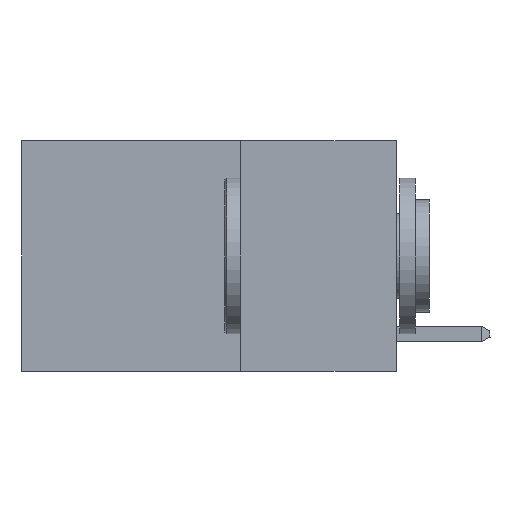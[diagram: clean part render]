
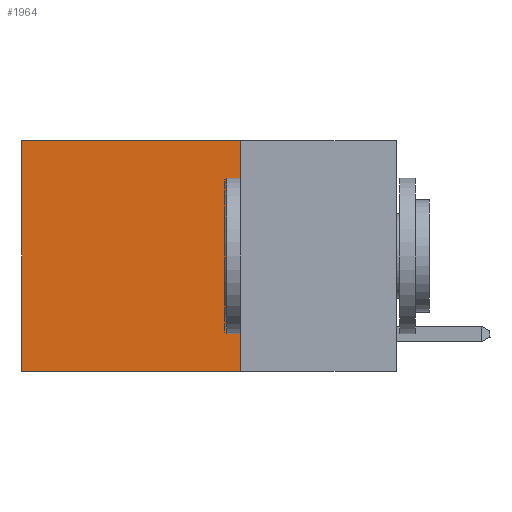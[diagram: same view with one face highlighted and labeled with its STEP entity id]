
A CAD part, left-side view. The second image highlights one B-rep face of the part: STEP entity #1964.
In plain terms, the highlighted planar face has unit normal (-1, 0, 0).
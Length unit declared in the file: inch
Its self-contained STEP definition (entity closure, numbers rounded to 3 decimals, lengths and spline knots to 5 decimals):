
#124 = LINE ( 'NONE', #7129, #6076 ) ;
#725 = VECTOR ( 'NONE', #1364, 39.37008 ) ;
#837 = EDGE_CURVE ( 'NONE', #999, #3835, #2540, .T. ) ;
#895 = DIRECTION ( 'NONE',  ( 0., 0., -1. ) ) ;
#999 = VERTEX_POINT ( 'NONE', #2601 ) ;
#1364 = DIRECTION ( 'NONE',  ( 0., 1., 0. ) ) ;
#1964 = ADVANCED_FACE ( 'NONE', ( #4877 ), #3511, .F. ) ;
#2136 = CARTESIAN_POINT ( 'NONE',  ( 0.2625, 0.25, -0.37 ) ) ;
#2264 = VERTEX_POINT ( 'NONE', #3410 ) ;
#2334 = CARTESIAN_POINT ( 'NONE',  ( 0.2625, 0.25, 0. ) ) ;
#2442 = DIRECTION ( 'NONE',  ( 0., 1., 0. ) ) ;
#2540 = LINE ( 'NONE', #2334, #4622 ) ;
#2601 = CARTESIAN_POINT ( 'NONE',  ( 0.2625, 0.25, 0. ) ) ;
#3062 = EDGE_CURVE ( 'NONE', #999, #2264, #9534, .T. ) ;
#3334 = CARTESIAN_POINT ( 'NONE',  ( 0.2625, 0.25, 0. ) ) ;
#3410 = CARTESIAN_POINT ( 'NONE',  ( 0.2625, 0.6, 0. ) ) ;
#3511 = PLANE ( 'NONE',  #5679 ) ;
#3623 = CARTESIAN_POINT ( 'NONE',  ( 0.2625, 0.6, -0.37 ) ) ;
#3731 = ORIENTED_EDGE ( 'NONE', *, *, #4255, .F. ) ;
#3835 = VERTEX_POINT ( 'NONE', #9492 ) ;
#3867 = ORIENTED_EDGE ( 'NONE', *, *, #837, .F. ) ;
#4100 = DIRECTION ( 'NONE',  ( 0., 0., -1. ) ) ;
#4255 = EDGE_CURVE ( 'NONE', #3835, #6592, #6164, .T. ) ;
#4622 = VECTOR ( 'NONE', #4100, 39.37008 ) ;
#4877 = FACE_OUTER_BOUND ( 'NONE', #6025, .T. ) ;
#5397 = ORIENTED_EDGE ( 'NONE', *, *, #3062, .T. ) ;
#5533 = CARTESIAN_POINT ( 'NONE',  ( 0.2625, 0.25, 0. ) ) ;
#5679 = AXIS2_PLACEMENT_3D ( 'NONE', #3334, #9868, #895 ) ;
#6025 = EDGE_LOOP ( 'NONE', ( #9340, #3731, #3867, #5397 ) ) ;
#6076 = VECTOR ( 'NONE', #6330, 39.37008 ) ;
#6164 = LINE ( 'NONE', #2136, #725 ) ;
#6330 = DIRECTION ( 'NONE',  ( 0., 0., -1. ) ) ;
#6592 = VERTEX_POINT ( 'NONE', #3623 ) ;
#7129 = CARTESIAN_POINT ( 'NONE',  ( 0.2625, 0.6, 0. ) ) ;
#7782 = EDGE_CURVE ( 'NONE', #2264, #6592, #124, .T. ) ;
#8412 = VECTOR ( 'NONE', #2442, 39.37008 ) ;
#9340 = ORIENTED_EDGE ( 'NONE', *, *, #7782, .T. ) ;
#9492 = CARTESIAN_POINT ( 'NONE',  ( 0.2625, 0.25, -0.37 ) ) ;
#9534 = LINE ( 'NONE', #5533, #8412 ) ;
#9868 = DIRECTION ( 'NONE',  ( 1., 0., 0. ) ) ;
